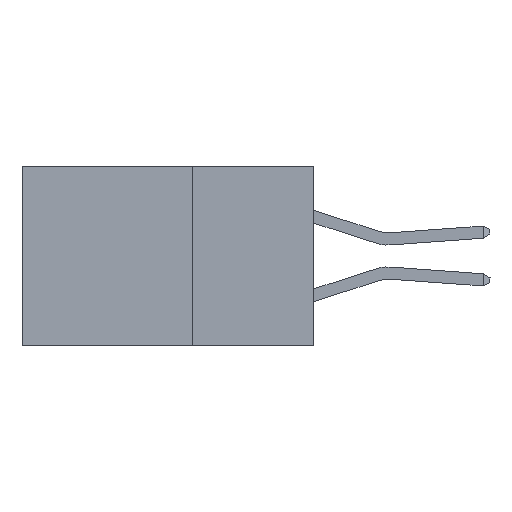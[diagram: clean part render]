
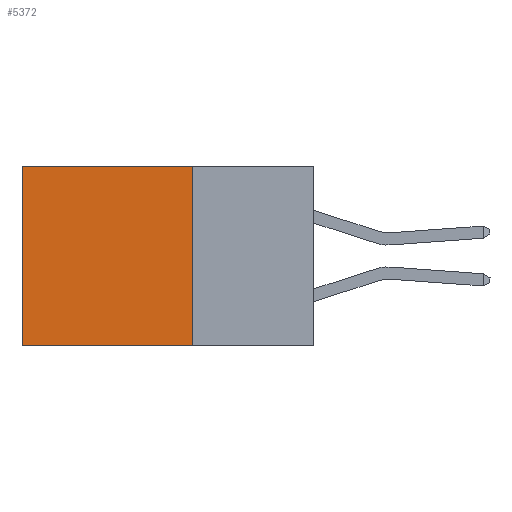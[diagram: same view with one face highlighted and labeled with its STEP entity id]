
A CAD part, left-side view. The second image highlights one B-rep face of the part: STEP entity #5372.
In plain terms, the highlighted planar face has unit normal (-1, 0, 0).
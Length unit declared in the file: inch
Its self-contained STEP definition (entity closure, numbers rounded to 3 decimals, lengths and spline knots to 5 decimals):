
#675 = LINE ( 'NONE', #21090, #22519 ) ;
#1315 = CARTESIAN_POINT ( 'NONE',  ( 0.2875, 0.25, -0.37 ) ) ;
#2244 = PLANE ( 'NONE',  #7587 ) ;
#2995 = ORIENTED_EDGE ( 'NONE', *, *, #13528, .T. ) ;
#3266 = VERTEX_POINT ( 'NONE', #23351 ) ;
#4527 = CARTESIAN_POINT ( 'NONE',  ( 0.2875, 0.25, 0. ) ) ;
#5372 = ADVANCED_FACE ( 'NONE', ( #31934 ), #2244, .F. ) ;
#5499 = DIRECTION ( 'NONE',  ( 1., 0., 0. ) ) ;
#5739 = EDGE_CURVE ( 'NONE', #11931, #8556, #675, .T. ) ;
#5770 = VECTOR ( 'NONE', #25106, 39.37008 ) ;
#6695 = EDGE_CURVE ( 'NONE', #28175, #8556, #23689, .T. ) ;
#7587 = AXIS2_PLACEMENT_3D ( 'NONE', #27711, #5499, #32066 ) ;
#8556 = VERTEX_POINT ( 'NONE', #16998 ) ;
#8746 = ORIENTED_EDGE ( 'NONE', *, *, #10205, .F. ) ;
#10205 = EDGE_CURVE ( 'NONE', #3266, #28175, #12085, .T. ) ;
#10357 = CARTESIAN_POINT ( 'NONE',  ( 0.2875, 0.6, 0. ) ) ;
#11372 = DIRECTION ( 'NONE',  ( 0., 1., 0. ) ) ;
#11931 = VERTEX_POINT ( 'NONE', #10357 ) ;
#12085 = LINE ( 'NONE', #4527, #5770 ) ;
#13145 = ORIENTED_EDGE ( 'NONE', *, *, #5739, .T. ) ;
#13528 = EDGE_CURVE ( 'NONE', #3266, #11931, #24390, .T. ) ;
#16998 = CARTESIAN_POINT ( 'NONE',  ( 0.2875, 0.6, -0.37 ) ) ;
#19338 = EDGE_LOOP ( 'NONE', ( #13145, #28366, #8746, #2995 ) ) ;
#21090 = CARTESIAN_POINT ( 'NONE',  ( 0.2875, 0.6, 0. ) ) ;
#21275 = CARTESIAN_POINT ( 'NONE',  ( 0.2875, 0.25, 0. ) ) ;
#22519 = VECTOR ( 'NONE', #30561, 39.37008 ) ;
#23351 = CARTESIAN_POINT ( 'NONE',  ( 0.2875, 0.25, 0. ) ) ;
#23689 = LINE ( 'NONE', #1315, #32270 ) ;
#23801 = DIRECTION ( 'NONE',  ( 0., 1., 0. ) ) ;
#24390 = LINE ( 'NONE', #21275, #30553 ) ;
#25106 = DIRECTION ( 'NONE',  ( 0., 0., -1. ) ) ;
#26393 = CARTESIAN_POINT ( 'NONE',  ( 0.2875, 0.25, -0.37 ) ) ;
#27711 = CARTESIAN_POINT ( 'NONE',  ( 0.2875, 0.25, 0. ) ) ;
#28175 = VERTEX_POINT ( 'NONE', #26393 ) ;
#28366 = ORIENTED_EDGE ( 'NONE', *, *, #6695, .F. ) ;
#30553 = VECTOR ( 'NONE', #23801, 39.37008 ) ;
#30561 = DIRECTION ( 'NONE',  ( 0., 0., -1. ) ) ;
#31934 = FACE_OUTER_BOUND ( 'NONE', #19338, .T. ) ;
#32066 = DIRECTION ( 'NONE',  ( 0., 0., -1. ) ) ;
#32270 = VECTOR ( 'NONE', #11372, 39.37008 ) ;
